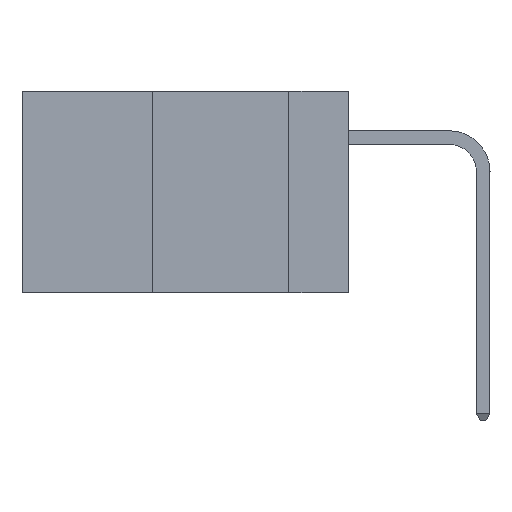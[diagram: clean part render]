
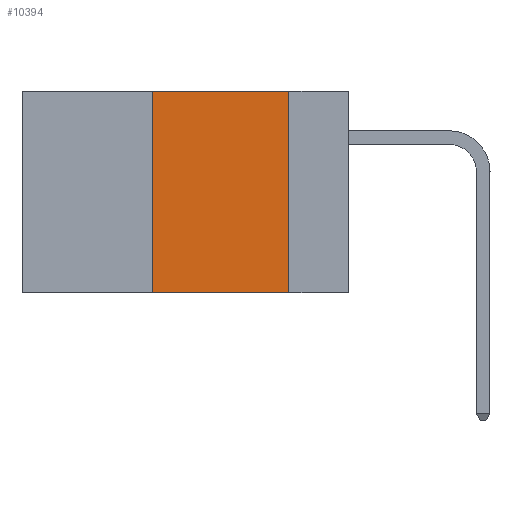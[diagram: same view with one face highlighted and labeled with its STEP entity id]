
A CAD part, left-side view. The second image highlights one B-rep face of the part: STEP entity #10394.
In plain terms, the highlighted planar face has unit normal (-1, 0, 0).
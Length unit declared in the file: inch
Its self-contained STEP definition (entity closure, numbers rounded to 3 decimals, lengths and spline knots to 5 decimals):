
#964 = PLANE ( 'NONE',  #22417 ) ;
#1166 = ORIENTED_EDGE ( 'NONE', *, *, #24894, .T. ) ;
#1300 = CARTESIAN_POINT ( 'NONE',  ( 0., 0.11, 0. ) ) ;
#2118 = LINE ( 'NONE', #3940, #24233 ) ;
#3940 = CARTESIAN_POINT ( 'NONE',  ( 0., 0.36, 0. ) ) ;
#4543 = CARTESIAN_POINT ( 'NONE',  ( 0., 0.36, -0.37 ) ) ;
#4555 = VECTOR ( 'NONE', #26335, 39.37008 ) ;
#5373 = VERTEX_POINT ( 'NONE', #25448 ) ;
#5728 = DIRECTION ( 'NONE',  ( 0., 0., -1. ) ) ;
#6005 = DIRECTION ( 'NONE',  ( 0., -1., 0. ) ) ;
#7045 = ORIENTED_EDGE ( 'NONE', *, *, #26619, .F. ) ;
#9094 = CARTESIAN_POINT ( 'NONE',  ( 0., 0.11, -0.37 ) ) ;
#9667 = DIRECTION ( 'NONE',  ( 1., 0., 0. ) ) ;
#10027 = CARTESIAN_POINT ( 'NONE',  ( 0., 0.6, -0.37 ) ) ;
#10394 = ADVANCED_FACE ( 'NONE', ( #17699 ), #964, .F. ) ;
#10777 = VECTOR ( 'NONE', #5728, 39.37008 ) ;
#11475 = ORIENTED_EDGE ( 'NONE', *, *, #18594, .F. ) ;
#14156 = LINE ( 'NONE', #1300, #10777 ) ;
#14184 = LINE ( 'NONE', #10027, #4555 ) ;
#14556 = VERTEX_POINT ( 'NONE', #26667 ) ;
#15805 = VECTOR ( 'NONE', #6005, 39.37008 ) ;
#16023 = CARTESIAN_POINT ( 'NONE',  ( 0., 0.6, 0. ) ) ;
#16503 = VERTEX_POINT ( 'NONE', #4543 ) ;
#17699 = FACE_OUTER_BOUND ( 'NONE', #27220, .T. ) ;
#17905 = ORIENTED_EDGE ( 'NONE', *, *, #21204, .F. ) ;
#18594 = EDGE_CURVE ( 'NONE', #5373, #14556, #24933, .T. ) ;
#20528 = CARTESIAN_POINT ( 'NONE',  ( 0., 0.6, 0. ) ) ;
#20938 = DIRECTION ( 'NONE',  ( 0., 0., 1. ) ) ;
#21204 = EDGE_CURVE ( 'NONE', #16503, #5373, #2118, .T. ) ;
#21825 = DIRECTION ( 'NONE',  ( 0., 0., -1. ) ) ;
#22169 = VERTEX_POINT ( 'NONE', #9094 ) ;
#22417 = AXIS2_PLACEMENT_3D ( 'NONE', #16023, #9667, #21825 ) ;
#24233 = VECTOR ( 'NONE', #20938, 39.37008 ) ;
#24894 = EDGE_CURVE ( 'NONE', #16503, #22169, #14184, .T. ) ;
#24933 = LINE ( 'NONE', #20528, #15805 ) ;
#25448 = CARTESIAN_POINT ( 'NONE',  ( 0., 0.36, 0. ) ) ;
#26335 = DIRECTION ( 'NONE',  ( 0., -1., 0. ) ) ;
#26619 = EDGE_CURVE ( 'NONE', #14556, #22169, #14156, .T. ) ;
#26667 = CARTESIAN_POINT ( 'NONE',  ( 0., 0.11, 0. ) ) ;
#27220 = EDGE_LOOP ( 'NONE', ( #7045, #11475, #17905, #1166 ) ) ;
